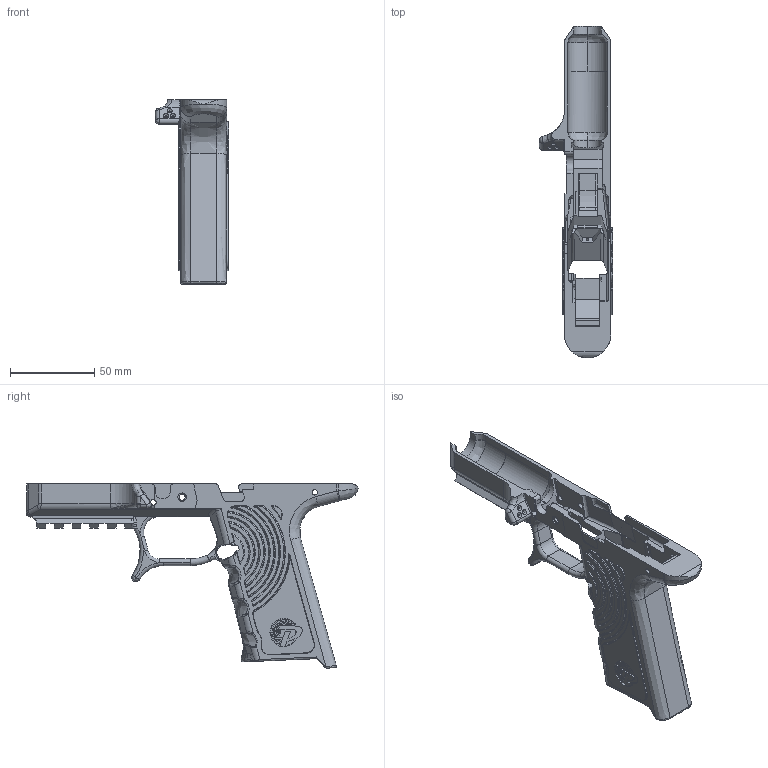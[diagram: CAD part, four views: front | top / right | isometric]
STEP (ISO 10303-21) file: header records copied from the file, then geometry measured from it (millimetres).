
FILE_DESCRIPTION(/* description */ (''),/* implementation_level */ '2;1');
FILE_NAME(/* name */ 'M&P 9 Assembly - MMMMandP.step',/* time_stamp */ '2021-12-01T00:21:08-05:00',/* author */ (''),/* organization */ (''),/* preprocessor_version */ 'ST-DEVELOPER v18.1',/* originating_system */ 'Autodesk Translation Framework v10.10.0.1391',/* authorisation */ '');
FILE_SCHEMA (('AUTOMOTIVE_DESIGN { 1 0 10303 214 3 1 1 }'));
Products named in the file (6): MMMMandP V2; M&P 9 Standard Length Slide - Picatinny v18; M&P 9 Reference v106; Frame; Fitment Section; Full-Size Magwell Body
Assembly tree (5 placements, depth 5):
  MMMMandP V2
    M&P 9 Standard Length Slide - Picatinny v18
      M&P 9 Reference v106
        Frame
          Fitment Section
          Full-Size Magwell Body
Bounding box: 43.6 x 197.48 x 109.57 mm (x, y, z)
Volume: 97534.9 mm3; surface area: 49870.5 mm2
Topology: 1 solids, 1 shells, 1375 faces, 3655 edges, 2300 vertices
Faces by surface type: bspline 644, plane 429, cylinder 228, torus 70, sphere 3, cone 1
Full cylindrical faces by diameter (mm): 1.5 x1, 3.18 x2, 3.361 x2, 3.55 x2, 5.1 x1
Entity records: 53967 total; most frequent: CARTESIAN_POINT 24773, ORIENTED_EDGE 7270, DIRECTION 4534, EDGE_CURVE 3635, VERTEX_POINT 2296, LINE 1588, VECTOR 1588, AXIS2_PLACEMENT_3D 1473
